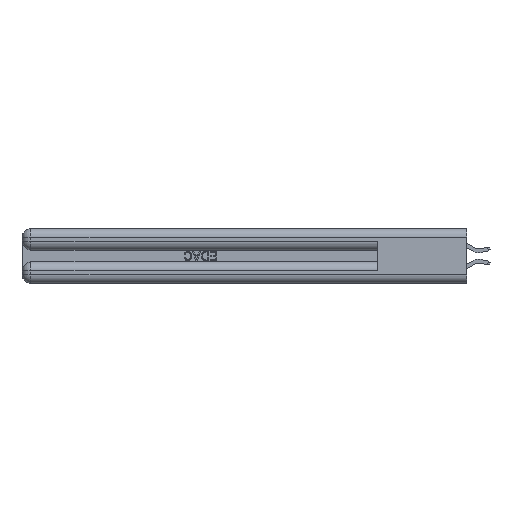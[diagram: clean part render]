
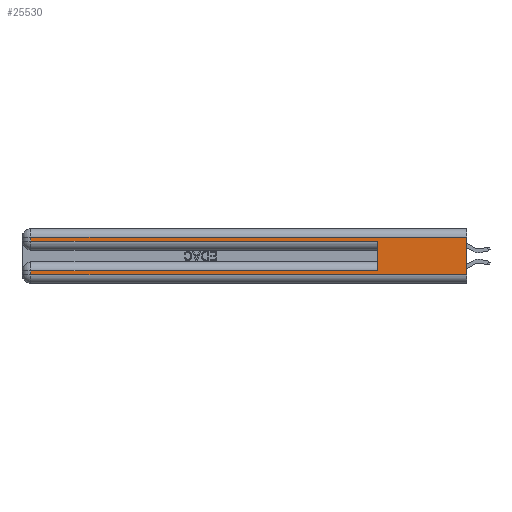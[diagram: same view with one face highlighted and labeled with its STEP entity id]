
A CAD part, left-side view. The second image highlights one B-rep face of the part: STEP entity #25530.
In plain terms, the highlighted planar face has unit normal (-1, 0, 0).
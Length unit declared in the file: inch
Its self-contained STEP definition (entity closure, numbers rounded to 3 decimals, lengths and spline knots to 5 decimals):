
#488 = DIRECTION ( 'NONE',  ( 1., 0., 0. ) ) ;
#1944 = LINE ( 'NONE', #23708, #17201 ) ;
#2484 = VECTOR ( 'NONE', #16207, 39.37008 ) ;
#2900 = CARTESIAN_POINT ( 'NONE',  ( 0., 0., 0.37 ) ) ;
#3363 = LINE ( 'NONE', #5795, #37038 ) ;
#4364 = DIRECTION ( 'NONE',  ( 0., 0., -1. ) ) ;
#5510 = DIRECTION ( 'NONE',  ( 0., 1., 0. ) ) ;
#5795 = CARTESIAN_POINT ( 'NONE',  ( 0., 0., 0.085 ) ) ;
#6080 = VERTEX_POINT ( 'NONE', #25749 ) ;
#6571 = DIRECTION ( 'NONE',  ( 0., -1., 0. ) ) ;
#6853 = VERTEX_POINT ( 'NONE', #38967 ) ;
#7238 = VECTOR ( 'NONE', #10794, 39.37008 ) ;
#8005 = CARTESIAN_POINT ( 'NONE',  ( 0., 0.6, 0.085 ) ) ;
#10045 = VERTEX_POINT ( 'NONE', #8005 ) ;
#10307 = ORIENTED_EDGE ( 'NONE', *, *, #42151, .F. ) ;
#10519 = CARTESIAN_POINT ( 'NONE',  ( 0., 0., 0.37 ) ) ;
#10794 = DIRECTION ( 'NONE',  ( 0., 0., -1. ) ) ;
#11924 = EDGE_CURVE ( 'NONE', #10045, #6853, #17194, .T. ) ;
#12150 = VECTOR ( 'NONE', #28415, 39.37008 ) ;
#12302 = VERTEX_POINT ( 'NONE', #33762 ) ;
#13226 = VERTEX_POINT ( 'NONE', #17141 ) ;
#13896 = ORIENTED_EDGE ( 'NONE', *, *, #18949, .T. ) ;
#13909 = CARTESIAN_POINT ( 'NONE',  ( 0., 2.94, 0.37 ) ) ;
#15692 = LINE ( 'NONE', #2900, #39188 ) ;
#15875 = LINE ( 'NONE', #13909, #7238 ) ;
#16207 = DIRECTION ( 'NONE',  ( 0., 1., 0. ) ) ;
#16430 = VERTEX_POINT ( 'NONE', #41321 ) ;
#16968 = ORIENTED_EDGE ( 'NONE', *, *, #29695, .T. ) ;
#17141 = CARTESIAN_POINT ( 'NONE',  ( 0., 2.94, 0.285 ) ) ;
#17194 = LINE ( 'NONE', #41559, #12150 ) ;
#17201 = VECTOR ( 'NONE', #4364, 39.37008 ) ;
#17414 = VECTOR ( 'NONE', #6571, 39.37008 ) ;
#18750 = ORIENTED_EDGE ( 'NONE', *, *, #11924, .F. ) ;
#18839 = EDGE_CURVE ( 'NONE', #16430, #12302, #29031, .T. ) ;
#18949 = EDGE_CURVE ( 'NONE', #12302, #13226, #1944, .T. ) ;
#19126 = ORIENTED_EDGE ( 'NONE', *, *, #30125, .T. ) ;
#23116 = LINE ( 'NONE', #33273, #41550 ) ;
#23318 = PLANE ( 'NONE',  #36399 ) ;
#23438 = VERTEX_POINT ( 'NONE', #24865 ) ;
#23708 = CARTESIAN_POINT ( 'NONE',  ( 0., 2.94, 0.37 ) ) ;
#24260 = CARTESIAN_POINT ( 'NONE',  ( 0., 0., 0.06 ) ) ;
#24865 = CARTESIAN_POINT ( 'NONE',  ( 0., 2.94, 0.085 ) ) ;
#24897 = ORIENTED_EDGE ( 'NONE', *, *, #18839, .T. ) ;
#25530 = ADVANCED_FACE ( 'NONE', ( #32782 ), #23318, .F. ) ;
#25749 = CARTESIAN_POINT ( 'NONE',  ( 0., 2.94, 0.06 ) ) ;
#25952 = DIRECTION ( 'NONE',  ( 0., 0., -1. ) ) ;
#26791 = ORIENTED_EDGE ( 'NONE', *, *, #39108, .T. ) ;
#27300 = EDGE_CURVE ( 'NONE', #10045, #23438, #3363, .T. ) ;
#28415 = DIRECTION ( 'NONE',  ( 0., 0., 1. ) ) ;
#29031 = LINE ( 'NONE', #39573, #2484 ) ;
#29695 = EDGE_CURVE ( 'NONE', #13226, #6853, #34796, .T. ) ;
#30125 = EDGE_CURVE ( 'NONE', #23438, #6080, #15875, .T. ) ;
#30281 = VERTEX_POINT ( 'NONE', #24260 ) ;
#32782 = FACE_OUTER_BOUND ( 'NONE', #40779, .T. ) ;
#33164 = DIRECTION ( 'NONE',  ( 0., 0., -1. ) ) ;
#33273 = CARTESIAN_POINT ( 'NONE',  ( 0., 0., 0.06 ) ) ;
#33762 = CARTESIAN_POINT ( 'NONE',  ( 0., 2.94, 0.31 ) ) ;
#34796 = LINE ( 'NONE', #41923, #17414 ) ;
#34868 = ORIENTED_EDGE ( 'NONE', *, *, #27300, .T. ) ;
#36399 = AXIS2_PLACEMENT_3D ( 'NONE', #10519, #488, #33164 ) ;
#37038 = VECTOR ( 'NONE', #5510, 39.37008 ) ;
#38967 = CARTESIAN_POINT ( 'NONE',  ( 0., 0.6, 0.285 ) ) ;
#39108 = EDGE_CURVE ( 'NONE', #6080, #30281, #23116, .T. ) ;
#39188 = VECTOR ( 'NONE', #25952, 39.37008 ) ;
#39410 = DIRECTION ( 'NONE',  ( 0., -1., 0. ) ) ;
#39573 = CARTESIAN_POINT ( 'NONE',  ( 0., 0., 0.31 ) ) ;
#40779 = EDGE_LOOP ( 'NONE', ( #10307, #24897, #13896, #16968, #18750, #34868, #19126, #26791 ) ) ;
#41321 = CARTESIAN_POINT ( 'NONE',  ( 0., 0., 0.31 ) ) ;
#41550 = VECTOR ( 'NONE', #39410, 39.37008 ) ;
#41559 = CARTESIAN_POINT ( 'NONE',  ( 0., 0.6, 0.145 ) ) ;
#41923 = CARTESIAN_POINT ( 'NONE',  ( 0., 0., 0.285 ) ) ;
#42151 = EDGE_CURVE ( 'NONE', #16430, #30281, #15692, .T. ) ;
